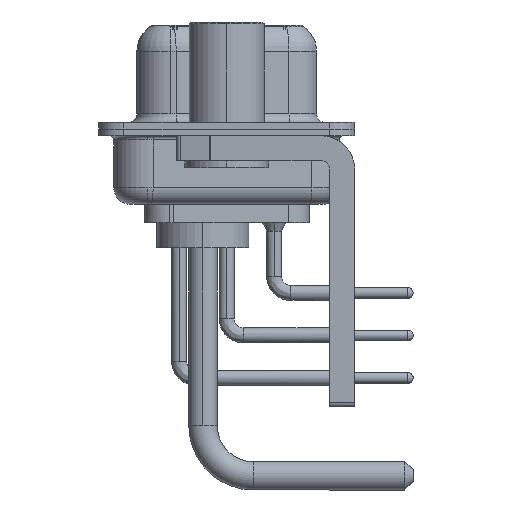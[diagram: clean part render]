
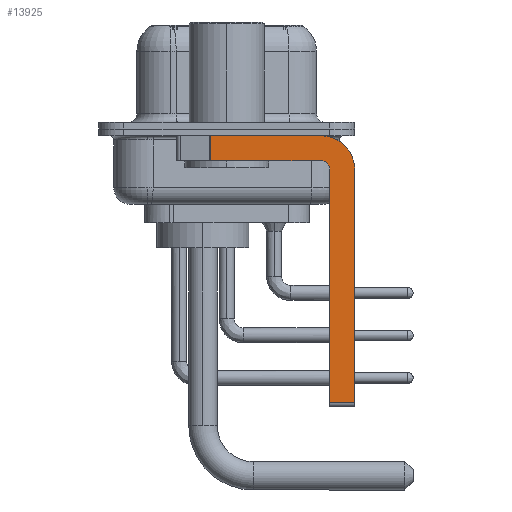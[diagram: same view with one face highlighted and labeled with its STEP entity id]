
A CAD part, left-side view. The second image highlights one B-rep face of the part: STEP entity #13925.
In plain terms, the highlighted planar face has unit normal (-1, 0, 0).
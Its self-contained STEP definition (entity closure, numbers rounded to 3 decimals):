
#520 = CARTESIAN_POINT ( 'NONE',  ( -2.9, -5.65, -1.9 ) ) ;
#838 = DIRECTION ( 'NONE',  ( 0., 1., 0. ) ) ;
#1627 = EDGE_CURVE ( 'NONE', #8453, #5341, #5370, .T. ) ;
#2625 = AXIS2_PLACEMENT_3D ( 'NONE', #23095, #28090, #22772 ) ;
#2642 = ORIENTED_EDGE ( 'NONE', *, *, #28228, .F. ) ;
#2752 = ORIENTED_EDGE ( 'NONE', *, *, #1627, .F. ) ;
#2941 = CARTESIAN_POINT ( 'NONE',  ( -2.9, -7.65, -16.35 ) ) ;
#3279 = VECTOR ( 'NONE', #25785, 1000. ) ;
#3454 = DIRECTION ( 'NONE',  ( -1., 0., 0. ) ) ;
#3716 = VERTEX_POINT ( 'NONE', #11979 ) ;
#4968 = ORIENTED_EDGE ( 'NONE', *, *, #10199, .F. ) ;
#5341 = VERTEX_POINT ( 'NONE', #18791 ) ;
#5370 = CIRCLE ( 'NONE', #23376, 0.5 ) ;
#5968 = DIRECTION ( 'NONE',  ( 0., 0., 1. ) ) ;
#5976 = CARTESIAN_POINT ( 'NONE',  ( -2.9, -5.65, -16.35 ) ) ;
#7885 = DIRECTION ( 'NONE',  ( 0., 0., -1. ) ) ;
#7948 = VERTEX_POINT ( 'NONE', #23300 ) ;
#8208 = DIRECTION ( 'NONE',  ( 1., 0., 0. ) ) ;
#8453 = VERTEX_POINT ( 'NONE', #25532 ) ;
#8556 = ORIENTED_EDGE ( 'NONE', *, *, #8787, .T. ) ;
#8787 = EDGE_CURVE ( 'NONE', #3716, #20020, #19234, .T. ) ;
#8898 = AXIS2_PLACEMENT_3D ( 'NONE', #22840, #8208, #7885 ) ;
#8906 = VECTOR ( 'NONE', #17215, 1000. ) ;
#8955 = EDGE_CURVE ( 'NONE', #5341, #20020, #22596, .T. ) ;
#9446 = ORIENTED_EDGE ( 'NONE', *, *, #17012, .T. ) ;
#9570 = CARTESIAN_POINT ( 'NONE',  ( -2.9, 0.978, -1.9 ) ) ;
#9657 = LINE ( 'NONE', #26569, #8906 ) ;
#9810 = VECTOR ( 'NONE', #31368, 1000. ) ;
#10199 = EDGE_CURVE ( 'NONE', #21786, #8453, #20775, .T. ) ;
#10590 = EDGE_LOOP ( 'NONE', ( #2642, #8556, #27453, #2752, #4968, #9446, #20031, #20357 ) ) ;
#10771 = EDGE_CURVE ( 'NONE', #7948, #16403, #21376, .T. ) ;
#10805 = CARTESIAN_POINT ( 'NONE',  ( -2.9, -6.15, -16.35 ) ) ;
#11049 = DIRECTION ( 'NONE',  ( 0., 0., 1. ) ) ;
#11296 = CARTESIAN_POINT ( 'NONE',  ( -2.9, -6.15, -16.6 ) ) ;
#11979 = CARTESIAN_POINT ( 'NONE',  ( -2.9, 0.978, -0.4 ) ) ;
#12943 = EDGE_CURVE ( 'NONE', #21634, #7948, #20646, .T. ) ;
#13182 = FACE_OUTER_BOUND ( 'NONE', #10590, .T. ) ;
#13308 = VECTOR ( 'NONE', #17450, 1000. ) ;
#13925 = ADVANCED_FACE ( 'NONE', ( #13182 ), #30253, .F. ) ;
#14361 = CARTESIAN_POINT ( 'NONE',  ( -2.9, -5.65, -0.4 ) ) ;
#14834 = VECTOR ( 'NONE', #838, 1000. ) ;
#16403 = VERTEX_POINT ( 'NONE', #2941 ) ;
#17012 = EDGE_CURVE ( 'NONE', #21786, #16403, #30932, .T. ) ;
#17215 = DIRECTION ( 'NONE',  ( 0., -1., 0. ) ) ;
#17450 = DIRECTION ( 'NONE',  ( 0., 0., -1. ) ) ;
#18791 = CARTESIAN_POINT ( 'NONE',  ( -2.9, -5.65, -1.9 ) ) ;
#19234 = LINE ( 'NONE', #9570, #13308 ) ;
#19555 = VECTOR ( 'NONE', #5968, 1000. ) ;
#20020 = VERTEX_POINT ( 'NONE', #22725 ) ;
#20031 = ORIENTED_EDGE ( 'NONE', *, *, #10771, .F. ) ;
#20357 = ORIENTED_EDGE ( 'NONE', *, *, #12943, .F. ) ;
#20646 = CIRCLE ( 'NONE', #2625, 2. ) ;
#20775 = LINE ( 'NONE', #11296, #19555 ) ;
#21376 = LINE ( 'NONE', #21687, #9810 ) ;
#21634 = VERTEX_POINT ( 'NONE', #14361 ) ;
#21687 = CARTESIAN_POINT ( 'NONE',  ( -2.9, -7.65, -2.4 ) ) ;
#21786 = VERTEX_POINT ( 'NONE', #10805 ) ;
#22596 = LINE ( 'NONE', #520, #14834 ) ;
#22725 = CARTESIAN_POINT ( 'NONE',  ( -2.9, 0.978, -1.9 ) ) ;
#22772 = DIRECTION ( 'NONE',  ( 0., 0., -1. ) ) ;
#22840 = CARTESIAN_POINT ( 'NONE',  ( -2.9, -5.65, -2.4 ) ) ;
#23095 = CARTESIAN_POINT ( 'NONE',  ( -2.9, -5.65, -2.4 ) ) ;
#23300 = CARTESIAN_POINT ( 'NONE',  ( -2.9, -7.65, -2.4 ) ) ;
#23376 = AXIS2_PLACEMENT_3D ( 'NONE', #25540, #3454, #11049 ) ;
#25532 = CARTESIAN_POINT ( 'NONE',  ( -2.9, -6.15, -2.4 ) ) ;
#25540 = CARTESIAN_POINT ( 'NONE',  ( -2.9, -5.65, -2.4 ) ) ;
#25785 = DIRECTION ( 'NONE',  ( 0., -1., 0. ) ) ;
#26569 = CARTESIAN_POINT ( 'NONE',  ( -2.9, 3., -0.4 ) ) ;
#27453 = ORIENTED_EDGE ( 'NONE', *, *, #8955, .F. ) ;
#28090 = DIRECTION ( 'NONE',  ( 1., 0., 0. ) ) ;
#28228 = EDGE_CURVE ( 'NONE', #3716, #21634, #9657, .T. ) ;
#30253 = PLANE ( 'NONE',  #8898 ) ;
#30932 = LINE ( 'NONE', #5976, #3279 ) ;
#31368 = DIRECTION ( 'NONE',  ( 0., 0., -1. ) ) ;
